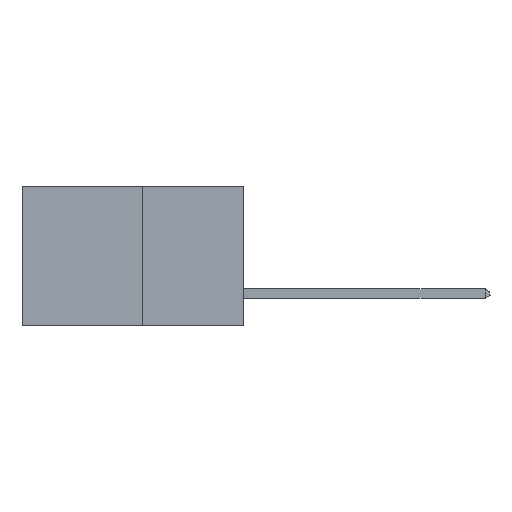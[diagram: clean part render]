
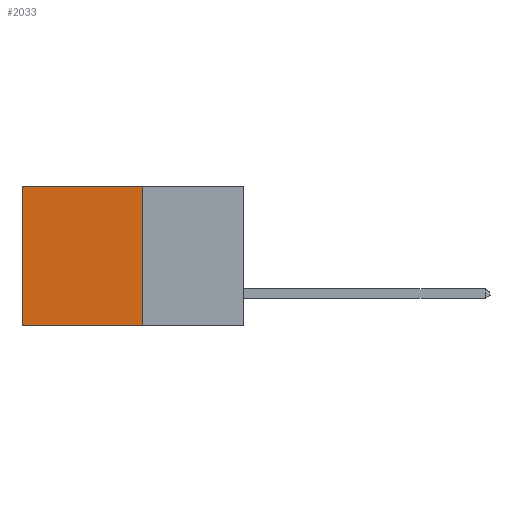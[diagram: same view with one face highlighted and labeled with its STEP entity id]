
A CAD part, left-side view. The second image highlights one B-rep face of the part: STEP entity #2033.
In plain terms, the highlighted planar face has unit normal (-1, 0, 0).
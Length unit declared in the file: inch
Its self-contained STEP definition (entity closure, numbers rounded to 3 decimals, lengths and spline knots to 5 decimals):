
#207 = VERTEX_POINT ( 'NONE', #16155 ) ;
#1182 = FACE_OUTER_BOUND ( 'NONE', #8251, .T. ) ;
#1412 = ORIENTED_EDGE ( 'NONE', *, *, #6634, .F. ) ;
#2033 = ADVANCED_FACE ( 'NONE', ( #1182 ), #15579, .F. ) ;
#2137 = CARTESIAN_POINT ( 'NONE',  ( 0.277, 0.27, -0.37 ) ) ;
#2484 = EDGE_CURVE ( 'NONE', #6204, #207, #18312, .T. ) ;
#2566 = EDGE_CURVE ( 'NONE', #4124, #14696, #20586, .T. ) ;
#2607 = ORIENTED_EDGE ( 'NONE', *, *, #11728, .T. ) ;
#4124 = VERTEX_POINT ( 'NONE', #9964 ) ;
#4823 = LINE ( 'NONE', #2137, #9266 ) ;
#6204 = VERTEX_POINT ( 'NONE', #19182 ) ;
#6634 = EDGE_CURVE ( 'NONE', #6204, #4124, #4823, .T. ) ;
#8251 = EDGE_LOOP ( 'NONE', ( #2607, #12848, #1412, #19056 ) ) ;
#8364 = CARTESIAN_POINT ( 'NONE',  ( 0.277, 0.59, -0.37 ) ) ;
#9266 = VECTOR ( 'NONE', #10457, 39.37008 ) ;
#9964 = CARTESIAN_POINT ( 'NONE',  ( 0.277, 0.27, -0.37 ) ) ;
#10457 = DIRECTION ( 'NONE',  ( 0., 0., -1. ) ) ;
#10894 = DIRECTION ( 'NONE',  ( 0., 1., 0. ) ) ;
#11290 = DIRECTION ( 'NONE',  ( 0., 1., 0. ) ) ;
#11728 = EDGE_CURVE ( 'NONE', #207, #14696, #21109, .T. ) ;
#11945 = CARTESIAN_POINT ( 'NONE',  ( 0.277, 0.27, -0.37 ) ) ;
#12848 = ORIENTED_EDGE ( 'NONE', *, *, #2566, .F. ) ;
#13800 = CARTESIAN_POINT ( 'NONE',  ( 0.277, 0.27, 0. ) ) ;
#14696 = VERTEX_POINT ( 'NONE', #20584 ) ;
#15028 = DIRECTION ( 'NONE',  ( 0., 0., -1. ) ) ;
#15481 = DIRECTION ( 'NONE',  ( 0., 0., -1. ) ) ;
#15521 = DIRECTION ( 'NONE',  ( 1., 0., 0. ) ) ;
#15553 = CARTESIAN_POINT ( 'NONE',  ( 0.277, 0.27, -0.37 ) ) ;
#15579 = PLANE ( 'NONE',  #15982 ) ;
#15982 = AXIS2_PLACEMENT_3D ( 'NONE', #15553, #15521, #15481 ) ;
#16155 = CARTESIAN_POINT ( 'NONE',  ( 0.277, 0.59, 0. ) ) ;
#16256 = VECTOR ( 'NONE', #10894, 39.37008 ) ;
#16783 = VECTOR ( 'NONE', #15028, 39.37008 ) ;
#17803 = VECTOR ( 'NONE', #11290, 39.37008 ) ;
#18312 = LINE ( 'NONE', #13800, #17803 ) ;
#19056 = ORIENTED_EDGE ( 'NONE', *, *, #2484, .T. ) ;
#19182 = CARTESIAN_POINT ( 'NONE',  ( 0.277, 0.27, 0. ) ) ;
#20584 = CARTESIAN_POINT ( 'NONE',  ( 0.277, 0.59, -0.37 ) ) ;
#20586 = LINE ( 'NONE', #11945, #16256 ) ;
#21109 = LINE ( 'NONE', #8364, #16783 ) ;
